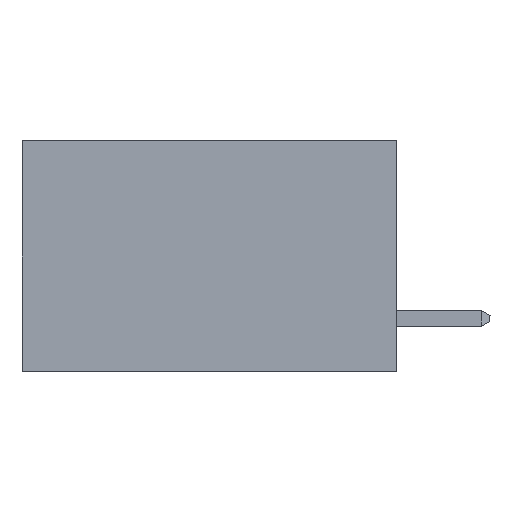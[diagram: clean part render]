
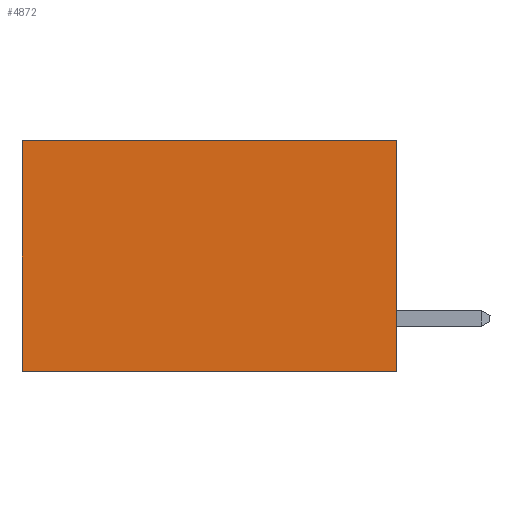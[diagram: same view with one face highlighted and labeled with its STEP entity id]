
A CAD part, left-side view. The second image highlights one B-rep face of the part: STEP entity #4872.
In plain terms, the highlighted planar face has unit normal (-1, 0, 0).
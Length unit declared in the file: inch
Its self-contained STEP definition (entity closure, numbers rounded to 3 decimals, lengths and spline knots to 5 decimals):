
#47 = CARTESIAN_POINT ( 'NONE',  ( 0.2615, 0.6, 0. ) ) ;
#92 = CARTESIAN_POINT ( 'NONE',  ( 0.2615, 0., -0.37 ) ) ;
#393 = VECTOR ( 'NONE', #4993, 39.37008 ) ;
#586 = EDGE_LOOP ( 'NONE', ( #11870, #7531, #12054, #9666 ) ) ;
#1049 = CARTESIAN_POINT ( 'NONE',  ( 0.2615, 0., -0.37 ) ) ;
#1710 = FACE_OUTER_BOUND ( 'NONE', #586, .T. ) ;
#2932 = DIRECTION ( 'NONE',  ( 0., 0., -1. ) ) ;
#3414 = VERTEX_POINT ( 'NONE', #8971 ) ;
#3809 = PLANE ( 'NONE',  #10553 ) ;
#4283 = CARTESIAN_POINT ( 'NONE',  ( 0.2615, 0.6, -0.37 ) ) ;
#4564 = DIRECTION ( 'NONE',  ( 0., 0., -1. ) ) ;
#4872 = ADVANCED_FACE ( 'NONE', ( #1710 ), #3809, .F. ) ;
#4993 = DIRECTION ( 'NONE',  ( 0., 1., 0. ) ) ;
#5010 = VECTOR ( 'NONE', #8951, 39.37008 ) ;
#5551 = CARTESIAN_POINT ( 'NONE',  ( 0.2615, 0., 0. ) ) ;
#6228 = EDGE_CURVE ( 'NONE', #9879, #10018, #6709, .T. ) ;
#6627 = EDGE_CURVE ( 'NONE', #8385, #3414, #10909, .T. ) ;
#6709 = LINE ( 'NONE', #92, #5010 ) ;
#7195 = CARTESIAN_POINT ( 'NONE',  ( 0.2615, 0., -0.37 ) ) ;
#7531 = ORIENTED_EDGE ( 'NONE', *, *, #9351, .F. ) ;
#8385 = VERTEX_POINT ( 'NONE', #47 ) ;
#8951 = DIRECTION ( 'NONE',  ( 0., 0., -1. ) ) ;
#8971 = CARTESIAN_POINT ( 'NONE',  ( 0.2615, 0.6, -0.37 ) ) ;
#9334 = DIRECTION ( 'NONE',  ( 1., 0., 0. ) ) ;
#9351 = EDGE_CURVE ( 'NONE', #10018, #3414, #13564, .T. ) ;
#9628 = CARTESIAN_POINT ( 'NONE',  ( 0.2615, 0., 0. ) ) ;
#9666 = ORIENTED_EDGE ( 'NONE', *, *, #10019, .T. ) ;
#9844 = DIRECTION ( 'NONE',  ( 0., 1., 0. ) ) ;
#9879 = VERTEX_POINT ( 'NONE', #9628 ) ;
#10018 = VERTEX_POINT ( 'NONE', #1049 ) ;
#10019 = EDGE_CURVE ( 'NONE', #9879, #8385, #10876, .T. ) ;
#10553 = AXIS2_PLACEMENT_3D ( 'NONE', #11662, #9334, #2932 ) ;
#10582 = VECTOR ( 'NONE', #4564, 39.37008 ) ;
#10614 = VECTOR ( 'NONE', #9844, 39.37008 ) ;
#10876 = LINE ( 'NONE', #5551, #10614 ) ;
#10909 = LINE ( 'NONE', #4283, #10582 ) ;
#11662 = CARTESIAN_POINT ( 'NONE',  ( 0.2615, 0., -0.37 ) ) ;
#11870 = ORIENTED_EDGE ( 'NONE', *, *, #6627, .T. ) ;
#12054 = ORIENTED_EDGE ( 'NONE', *, *, #6228, .F. ) ;
#13564 = LINE ( 'NONE', #7195, #393 ) ;
